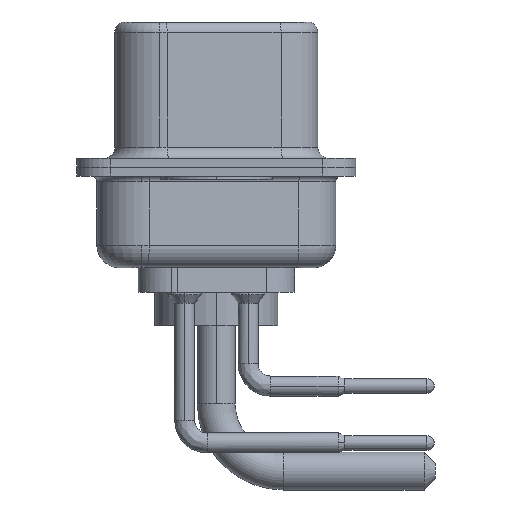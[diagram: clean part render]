
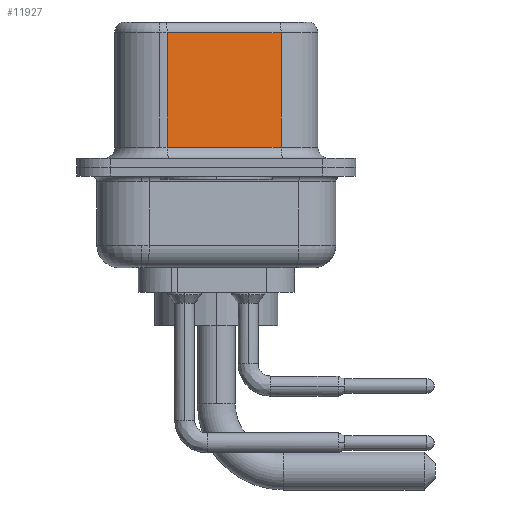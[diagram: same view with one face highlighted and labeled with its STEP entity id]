
A CAD part, left-side view. The second image highlights one B-rep face of the part: STEP entity #11927.
In plain terms, the highlighted planar face has unit normal (-0.985, -0.174, 0).
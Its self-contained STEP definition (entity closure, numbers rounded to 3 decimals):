
#40 = VECTOR ( 'NONE', #12457, 1000. ) ;
#94 = VERTEX_POINT ( 'NONE', #3978 ) ;
#250 = CARTESIAN_POINT ( 'NONE',  ( 3.68, 2.203, 0.9 ) ) ;
#885 = CARTESIAN_POINT ( 'NONE',  ( 4.58, -2.897, 6.52 ) ) ;
#935 = CARTESIAN_POINT ( 'NONE',  ( 4.58, -2.897, 6.52 ) ) ;
#1051 = EDGE_CURVE ( 'NONE', #13921, #14617, #17511, .T. ) ;
#1666 = CARTESIAN_POINT ( 'NONE',  ( 4.58, -2.897, 6.02 ) ) ;
#1732 = VERTEX_POINT ( 'NONE', #8384 ) ;
#2161 = LINE ( 'NONE', #16983, #16120 ) ;
#2204 = LINE ( 'NONE', #885, #4990 ) ;
#3391 = ORIENTED_EDGE ( 'NONE', *, *, #4112, .T. ) ;
#3978 = CARTESIAN_POINT ( 'NONE',  ( 4.58, -2.897, 6.02 ) ) ;
#4023 = CARTESIAN_POINT ( 'NONE',  ( 3.68, 2.203, 6.52 ) ) ;
#4112 = EDGE_CURVE ( 'NONE', #14617, #1732, #2161, .T. ) ;
#4546 = ORIENTED_EDGE ( 'NONE', *, *, #9837, .F. ) ;
#4990 = VECTOR ( 'NONE', #10384, 1000. ) ;
#6286 = VECTOR ( 'NONE', #8155, 1000. ) ;
#7586 = FACE_OUTER_BOUND ( 'NONE', #8472, .T. ) ;
#8155 = DIRECTION ( 'NONE',  ( -0.174, 0.985, 0. ) ) ;
#8290 = ORIENTED_EDGE ( 'NONE', *, *, #12398, .T. ) ;
#8384 = CARTESIAN_POINT ( 'NONE',  ( 4.58, -2.897, 0.9 ) ) ;
#8472 = EDGE_LOOP ( 'NONE', ( #4546, #8290, #11664, #3391 ) ) ;
#9837 = EDGE_CURVE ( 'NONE', #94, #1732, #2204, .T. ) ;
#10384 = DIRECTION ( 'NONE',  ( 0., 0., -1. ) ) ;
#10945 = DIRECTION ( 'NONE',  ( -0.174, 0.985, 0. ) ) ;
#11664 = ORIENTED_EDGE ( 'NONE', *, *, #1051, .T. ) ;
#11927 = ADVANCED_FACE ( 'NONE', ( #7586 ), #13016, .F. ) ;
#12398 = EDGE_CURVE ( 'NONE', #94, #13921, #16323, .T. ) ;
#12457 = DIRECTION ( 'NONE',  ( 0., 0., -1. ) ) ;
#13016 = PLANE ( 'NONE',  #16471 ) ;
#13921 = VERTEX_POINT ( 'NONE', #15989 ) ;
#14612 = DIRECTION ( 'NONE',  ( 0.174, -0.985, 0. ) ) ;
#14617 = VERTEX_POINT ( 'NONE', #250 ) ;
#14786 = DIRECTION ( 'NONE',  ( 0.985, 0.174, 0. ) ) ;
#15989 = CARTESIAN_POINT ( 'NONE',  ( 3.68, 2.203, 6.02 ) ) ;
#16120 = VECTOR ( 'NONE', #14612, 1000. ) ;
#16323 = LINE ( 'NONE', #1666, #6286 ) ;
#16471 = AXIS2_PLACEMENT_3D ( 'NONE', #935, #14786, #10945 ) ;
#16983 = CARTESIAN_POINT ( 'NONE',  ( 4.58, -2.897, 0.9 ) ) ;
#17511 = LINE ( 'NONE', #4023, #40 ) ;
